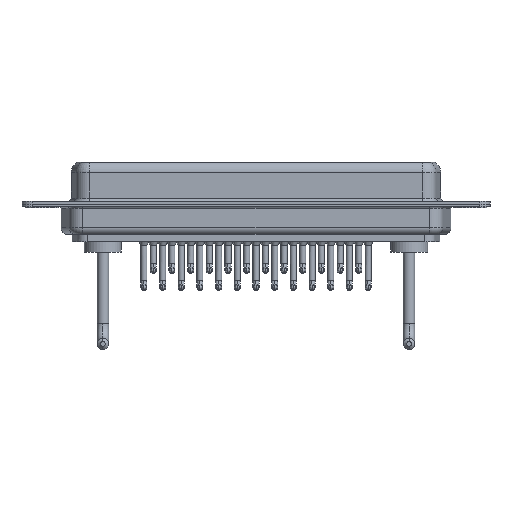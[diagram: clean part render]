
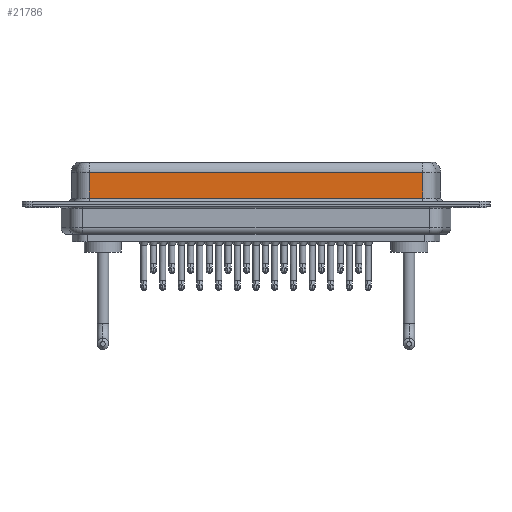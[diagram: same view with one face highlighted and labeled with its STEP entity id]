
A CAD part, front view. The second image highlights one B-rep face of the part: STEP entity #21786.
In plain terms, the highlighted planar face has unit normal (0, -1, 0).
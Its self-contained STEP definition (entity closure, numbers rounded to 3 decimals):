
#1336 = VECTOR ( 'NONE', #12439, 1000. ) ;
#1754 = FACE_OUTER_BOUND ( 'NONE', #9329, .T. ) ;
#2033 = DIRECTION ( 'NONE',  ( -1., 0., 0. ) ) ;
#3518 = CARTESIAN_POINT ( 'NONE',  ( 56.462, -3.95, 0.9 ) ) ;
#3676 = VECTOR ( 'NONE', #9067, 1000. ) ;
#3884 = CARTESIAN_POINT ( 'NONE',  ( 7.038, -3.95, 6.4 ) ) ;
#4185 = CARTESIAN_POINT ( 'NONE',  ( 7.038, -3.95, 4.65 ) ) ;
#5082 = EDGE_CURVE ( 'NONE', #17936, #17481, #16537, .T. ) ;
#5515 = LINE ( 'NONE', #17987, #14798 ) ;
#5943 = EDGE_CURVE ( 'NONE', #16115, #17936, #7160, .T. ) ;
#6005 = EDGE_CURVE ( 'NONE', #19660, #16115, #5515, .T. ) ;
#7160 = LINE ( 'NONE', #3884, #11816 ) ;
#7217 = LINE ( 'NONE', #10814, #3676 ) ;
#7571 = CARTESIAN_POINT ( 'NONE',  ( 56.462, -3.95, 0.9 ) ) ;
#8598 = ORIENTED_EDGE ( 'NONE', *, *, #5082, .T. ) ;
#8859 = DIRECTION ( 'NONE',  ( 0., 0., 1. ) ) ;
#9067 = DIRECTION ( 'NONE',  ( 0., 0., -1. ) ) ;
#9329 = EDGE_LOOP ( 'NONE', ( #16681, #17344, #20873, #8598 ) ) ;
#10636 = DIRECTION ( 'NONE',  ( 0., 0., -1. ) ) ;
#10814 = CARTESIAN_POINT ( 'NONE',  ( 56.462, -3.95, 6.4 ) ) ;
#11816 = VECTOR ( 'NONE', #10636, 1000. ) ;
#12243 = CARTESIAN_POINT ( 'NONE',  ( 56.462, -3.95, 6.4 ) ) ;
#12344 = CARTESIAN_POINT ( 'NONE',  ( 7.038, -3.95, 0.9 ) ) ;
#12439 = DIRECTION ( 'NONE',  ( 1., 0., 0. ) ) ;
#14111 = PLANE ( 'NONE',  #15943 ) ;
#14798 = VECTOR ( 'NONE', #2033, 1000. ) ;
#14973 = CARTESIAN_POINT ( 'NONE',  ( 56.462, -3.95, 4.65 ) ) ;
#15943 = AXIS2_PLACEMENT_3D ( 'NONE', #12243, #22841, #8859 ) ;
#16115 = VERTEX_POINT ( 'NONE', #4185 ) ;
#16537 = LINE ( 'NONE', #7571, #1336 ) ;
#16681 = ORIENTED_EDGE ( 'NONE', *, *, #22204, .F. ) ;
#17344 = ORIENTED_EDGE ( 'NONE', *, *, #6005, .T. ) ;
#17481 = VERTEX_POINT ( 'NONE', #3518 ) ;
#17936 = VERTEX_POINT ( 'NONE', #12344 ) ;
#17987 = CARTESIAN_POINT ( 'NONE',  ( 56.462, -3.95, 4.65 ) ) ;
#19660 = VERTEX_POINT ( 'NONE', #14973 ) ;
#20873 = ORIENTED_EDGE ( 'NONE', *, *, #5943, .T. ) ;
#21786 = ADVANCED_FACE ( 'NONE', ( #1754 ), #14111, .F. ) ;
#22204 = EDGE_CURVE ( 'NONE', #19660, #17481, #7217, .T. ) ;
#22841 = DIRECTION ( 'NONE',  ( 0., 1., 0. ) ) ;
